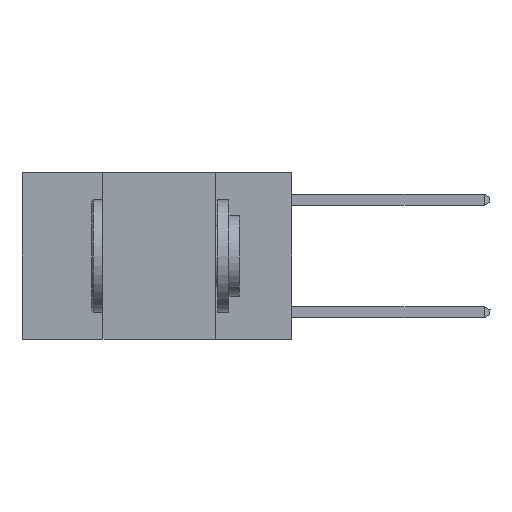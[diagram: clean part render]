
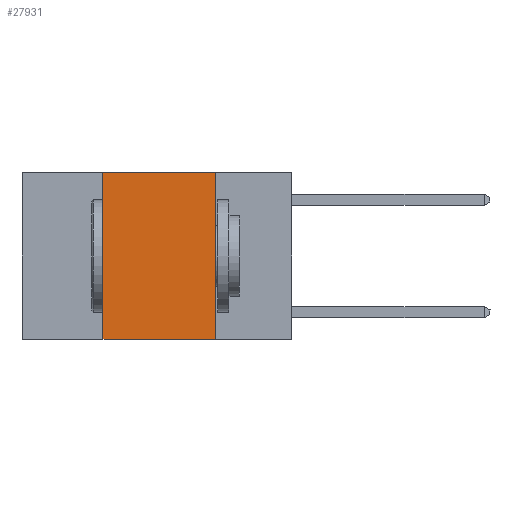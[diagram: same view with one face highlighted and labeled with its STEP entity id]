
A CAD part, left-side view. The second image highlights one B-rep face of the part: STEP entity #27931.
In plain terms, the highlighted planar face has unit normal (-1, 0, 0).
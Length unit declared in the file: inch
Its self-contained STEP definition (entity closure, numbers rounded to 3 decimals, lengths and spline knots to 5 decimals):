
#100 = CARTESIAN_POINT ( 'NONE',  ( 0., 0.42, 0. ) ) ;
#880 = VERTEX_POINT ( 'NONE', #5897 ) ;
#1026 = LINE ( 'NONE', #31392, #30838 ) ;
#1291 = VERTEX_POINT ( 'NONE', #30643 ) ;
#5897 = CARTESIAN_POINT ( 'NONE',  ( 0., 0.42, 0. ) ) ;
#6110 = PLANE ( 'NONE',  #9067 ) ;
#6310 = LINE ( 'NONE', #31872, #22411 ) ;
#6668 = VECTOR ( 'NONE', #20632, 39.37008 ) ;
#8091 = ORIENTED_EDGE ( 'NONE', *, *, #11442, .F. ) ;
#8665 = DIRECTION ( 'NONE',  ( 0., 0., -1. ) ) ;
#9067 = AXIS2_PLACEMENT_3D ( 'NONE', #31332, #11244, #18731 ) ;
#11244 = DIRECTION ( 'NONE',  ( 1., 0., 0. ) ) ;
#11442 = EDGE_CURVE ( 'NONE', #1291, #880, #28151, .T. ) ;
#12406 = LINE ( 'NONE', #22534, #6668 ) ;
#12827 = VERTEX_POINT ( 'NONE', #14923 ) ;
#13335 = ORIENTED_EDGE ( 'NONE', *, *, #27548, .T. ) ;
#14247 = ORIENTED_EDGE ( 'NONE', *, *, #27117, .F. ) ;
#14654 = EDGE_CURVE ( 'NONE', #880, #12827, #12406, .T. ) ;
#14923 = CARTESIAN_POINT ( 'NONE',  ( 0., 0.17, 0. ) ) ;
#15562 = DIRECTION ( 'NONE',  ( 0., 0., 1. ) ) ;
#18392 = VECTOR ( 'NONE', #15562, 39.37008 ) ;
#18731 = DIRECTION ( 'NONE',  ( 0., 0., -1. ) ) ;
#20632 = DIRECTION ( 'NONE',  ( 0., -1., 0. ) ) ;
#22411 = VECTOR ( 'NONE', #26550, 39.37008 ) ;
#22534 = CARTESIAN_POINT ( 'NONE',  ( 0., 0.6, 0. ) ) ;
#23615 = EDGE_LOOP ( 'NONE', ( #14247, #25585, #8091, #13335 ) ) ;
#23707 = CARTESIAN_POINT ( 'NONE',  ( 0., 0.17, -0.37 ) ) ;
#24245 = VERTEX_POINT ( 'NONE', #23707 ) ;
#25585 = ORIENTED_EDGE ( 'NONE', *, *, #14654, .F. ) ;
#26506 = FACE_OUTER_BOUND ( 'NONE', #23615, .T. ) ;
#26550 = DIRECTION ( 'NONE',  ( 0., -1., 0. ) ) ;
#27117 = EDGE_CURVE ( 'NONE', #12827, #24245, #1026, .T. ) ;
#27548 = EDGE_CURVE ( 'NONE', #1291, #24245, #6310, .T. ) ;
#27931 = ADVANCED_FACE ( 'NONE', ( #26506 ), #6110, .F. ) ;
#28151 = LINE ( 'NONE', #100, #18392 ) ;
#30643 = CARTESIAN_POINT ( 'NONE',  ( 0., 0.42, -0.37 ) ) ;
#30838 = VECTOR ( 'NONE', #8665, 39.37008 ) ;
#31332 = CARTESIAN_POINT ( 'NONE',  ( 0., 0.6, 0. ) ) ;
#31392 = CARTESIAN_POINT ( 'NONE',  ( 0., 0.17, 0. ) ) ;
#31872 = CARTESIAN_POINT ( 'NONE',  ( 0., 0.6, -0.37 ) ) ;
